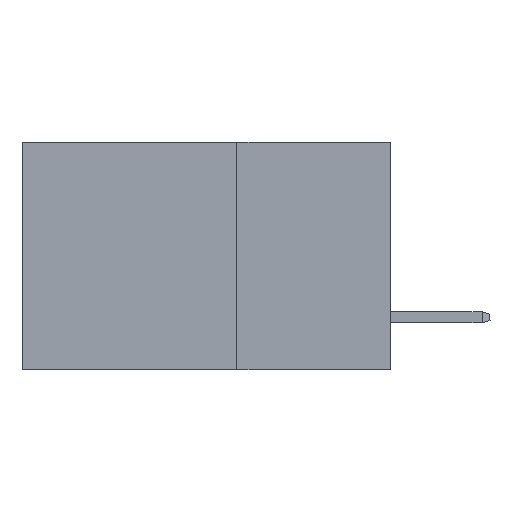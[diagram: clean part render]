
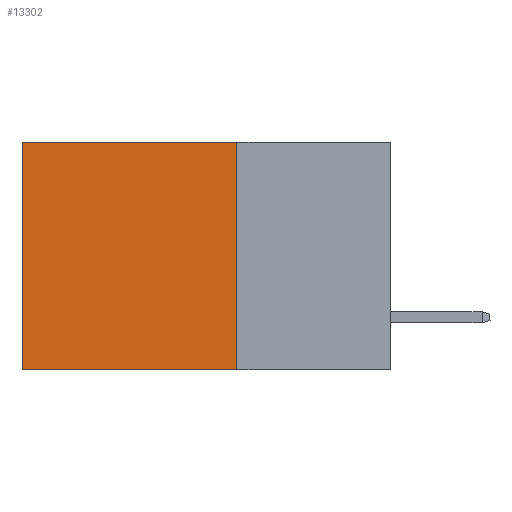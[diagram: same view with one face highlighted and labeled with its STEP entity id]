
A CAD part, left-side view. The second image highlights one B-rep face of the part: STEP entity #13302.
In plain terms, the highlighted planar face has unit normal (-1, 0, 0).
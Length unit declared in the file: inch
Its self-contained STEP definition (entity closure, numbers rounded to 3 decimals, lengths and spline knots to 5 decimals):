
#604 = EDGE_CURVE ( 'NONE', #2306, #11244, #10990, .T. ) ;
#779 = LINE ( 'NONE', #12805, #13993 ) ;
#1073 = CARTESIAN_POINT ( 'NONE',  ( 0.2875, 0.25, 0. ) ) ;
#1172 = CARTESIAN_POINT ( 'NONE',  ( 0.2875, 0.25, -0.37 ) ) ;
#1211 = EDGE_CURVE ( 'NONE', #1488, #2306, #779, .T. ) ;
#1488 = VERTEX_POINT ( 'NONE', #14387 ) ;
#1495 = ORIENTED_EDGE ( 'NONE', *, *, #1211, .T. ) ;
#1497 = ORIENTED_EDGE ( 'NONE', *, *, #3579, .F. ) ;
#2306 = VERTEX_POINT ( 'NONE', #4694 ) ;
#2360 = CARTESIAN_POINT ( 'NONE',  ( 0.2875, 0.6, 0. ) ) ;
#2500 = VECTOR ( 'NONE', #12297, 39.37008 ) ;
#2832 = DIRECTION ( 'NONE',  ( 1., 0., 0. ) ) ;
#2848 = ORIENTED_EDGE ( 'NONE', *, *, #10769, .F. ) ;
#3516 = VECTOR ( 'NONE', #5759, 39.37008 ) ;
#3579 = EDGE_CURVE ( 'NONE', #1488, #6522, #4392, .T. ) ;
#3850 = CARTESIAN_POINT ( 'NONE',  ( 0.2875, 0.25, 0. ) ) ;
#4392 = LINE ( 'NONE', #1073, #3516 ) ;
#4694 = CARTESIAN_POINT ( 'NONE',  ( 0.2875, 0.6, 0. ) ) ;
#5759 = DIRECTION ( 'NONE',  ( 0., 0., -1. ) ) ;
#6522 = VERTEX_POINT ( 'NONE', #1172 ) ;
#7006 = AXIS2_PLACEMENT_3D ( 'NONE', #3850, #2832, #14206 ) ;
#7311 = PLANE ( 'NONE',  #7006 ) ;
#7635 = EDGE_LOOP ( 'NONE', ( #10698, #2848, #1497, #1495 ) ) ;
#10020 = CARTESIAN_POINT ( 'NONE',  ( 0.2875, 0.25, -0.37 ) ) ;
#10411 = DIRECTION ( 'NONE',  ( 0., 1., 0. ) ) ;
#10487 = LINE ( 'NONE', #10020, #2500 ) ;
#10698 = ORIENTED_EDGE ( 'NONE', *, *, #604, .T. ) ;
#10769 = EDGE_CURVE ( 'NONE', #6522, #11244, #10487, .T. ) ;
#10940 = FACE_OUTER_BOUND ( 'NONE', #7635, .T. ) ;
#10990 = LINE ( 'NONE', #2360, #14926 ) ;
#11244 = VERTEX_POINT ( 'NONE', #12925 ) ;
#12297 = DIRECTION ( 'NONE',  ( 0., 1., 0. ) ) ;
#12805 = CARTESIAN_POINT ( 'NONE',  ( 0.2875, 0.25, 0. ) ) ;
#12925 = CARTESIAN_POINT ( 'NONE',  ( 0.2875, 0.6, -0.37 ) ) ;
#13302 = ADVANCED_FACE ( 'NONE', ( #10940 ), #7311, .F. ) ;
#13993 = VECTOR ( 'NONE', #10411, 39.37008 ) ;
#14206 = DIRECTION ( 'NONE',  ( 0., 0., -1. ) ) ;
#14387 = CARTESIAN_POINT ( 'NONE',  ( 0.2875, 0.25, 0. ) ) ;
#14926 = VECTOR ( 'NONE', #14969, 39.37008 ) ;
#14969 = DIRECTION ( 'NONE',  ( 0., 0., -1. ) ) ;
